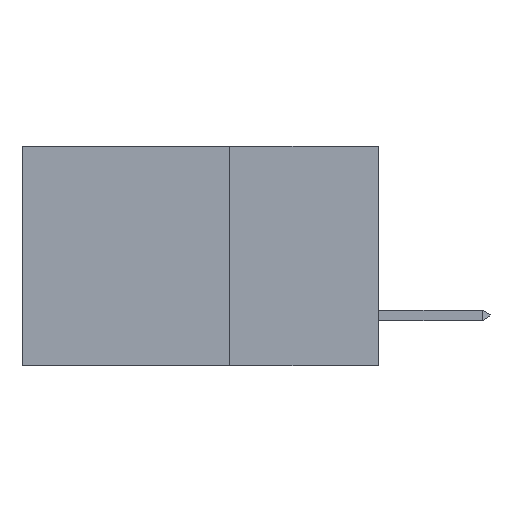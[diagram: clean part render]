
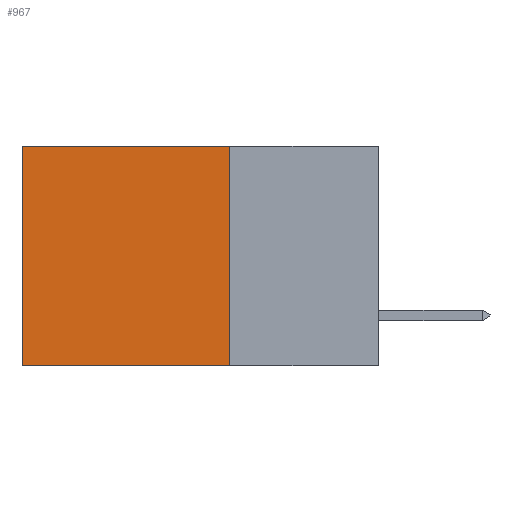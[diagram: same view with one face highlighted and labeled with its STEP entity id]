
A CAD part, left-side view. The second image highlights one B-rep face of the part: STEP entity #967.
In plain terms, the highlighted planar face has unit normal (-1, 0, 0).
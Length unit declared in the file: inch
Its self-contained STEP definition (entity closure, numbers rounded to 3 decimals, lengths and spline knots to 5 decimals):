
#710 = EDGE_CURVE ( 'NONE', #22908, #23629, #9976, .T. ) ;
#929 = CARTESIAN_POINT ( 'NONE',  ( 0.298, 0.25, 0. ) ) ;
#967 = ADVANCED_FACE ( 'NONE', ( #22932 ), #23608, .F. ) ;
#1744 = VECTOR ( 'NONE', #17343, 39.37008 ) ;
#2443 = CARTESIAN_POINT ( 'NONE',  ( 0.298, 0.25, 0. ) ) ;
#2904 = LINE ( 'NONE', #929, #11262 ) ;
#3159 = DIRECTION ( 'NONE',  ( 0., 0., -1. ) ) ;
#3392 = CARTESIAN_POINT ( 'NONE',  ( 0.298, 0.25, -0.37 ) ) ;
#4387 = ORIENTED_EDGE ( 'NONE', *, *, #710, .T. ) ;
#5075 = CARTESIAN_POINT ( 'NONE',  ( 0.298, 0.6, -0.37 ) ) ;
#6358 = VERTEX_POINT ( 'NONE', #5075 ) ;
#6819 = CARTESIAN_POINT ( 'NONE',  ( 0.298, 0.25, 0. ) ) ;
#8178 = AXIS2_PLACEMENT_3D ( 'NONE', #6819, #8979, #19458 ) ;
#8953 = CARTESIAN_POINT ( 'NONE',  ( 0.298, 0.6, 0. ) ) ;
#8979 = DIRECTION ( 'NONE',  ( 1., 0., 0. ) ) ;
#9693 = DIRECTION ( 'NONE',  ( 0., 1., 0. ) ) ;
#9853 = CARTESIAN_POINT ( 'NONE',  ( 0.298, 0.6, 0. ) ) ;
#9976 = LINE ( 'NONE', #26817, #23628 ) ;
#10022 = ORIENTED_EDGE ( 'NONE', *, *, #26974, .T. ) ;
#11193 = EDGE_CURVE ( 'NONE', #22908, #26174, #2904, .T. ) ;
#11262 = VECTOR ( 'NONE', #3159, 39.37008 ) ;
#11395 = ORIENTED_EDGE ( 'NONE', *, *, #11193, .F. ) ;
#13109 = CARTESIAN_POINT ( 'NONE',  ( 0.298, 0.25, -0.37 ) ) ;
#13194 = DIRECTION ( 'NONE',  ( 0., 1., 0. ) ) ;
#17343 = DIRECTION ( 'NONE',  ( 0., 0., -1. ) ) ;
#18049 = EDGE_CURVE ( 'NONE', #26174, #6358, #18888, .T. ) ;
#18888 = LINE ( 'NONE', #13109, #25260 ) ;
#19458 = DIRECTION ( 'NONE',  ( 0., 0., -1. ) ) ;
#22443 = ORIENTED_EDGE ( 'NONE', *, *, #18049, .F. ) ;
#22537 = EDGE_LOOP ( 'NONE', ( #10022, #22443, #11395, #4387 ) ) ;
#22908 = VERTEX_POINT ( 'NONE', #2443 ) ;
#22932 = FACE_OUTER_BOUND ( 'NONE', #22537, .T. ) ;
#23608 = PLANE ( 'NONE',  #8178 ) ;
#23629 = VERTEX_POINT ( 'NONE', #9853 ) ;
#23628 = VECTOR ( 'NONE', #9693, 39.37008 ) ;
#25260 = VECTOR ( 'NONE', #13194, 39.37008 ) ;
#26174 = VERTEX_POINT ( 'NONE', #3392 ) ;
#26817 = CARTESIAN_POINT ( 'NONE',  ( 0.298, 0.25, 0. ) ) ;
#26974 = EDGE_CURVE ( 'NONE', #23629, #6358, #27486, .T. ) ;
#27486 = LINE ( 'NONE', #8953, #1744 ) ;
